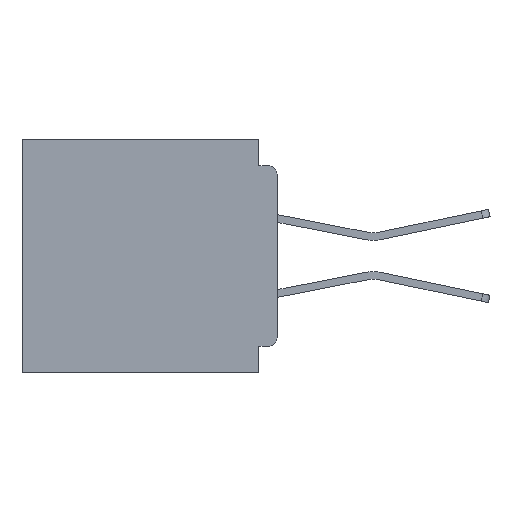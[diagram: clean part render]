
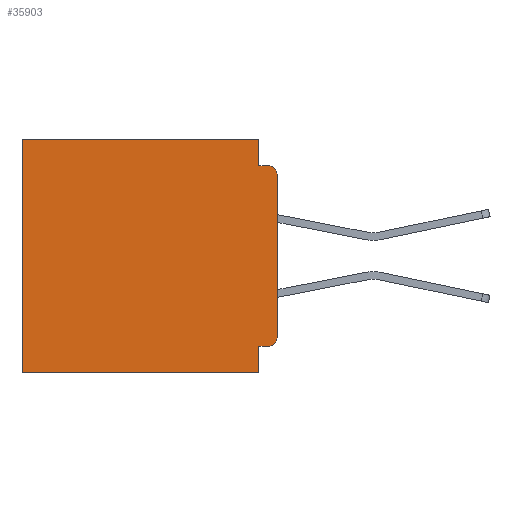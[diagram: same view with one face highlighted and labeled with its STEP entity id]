
A CAD part, left-side view. The second image highlights one B-rep face of the part: STEP entity #35903.
In plain terms, the highlighted planar face has unit normal (-1, 0, 0).
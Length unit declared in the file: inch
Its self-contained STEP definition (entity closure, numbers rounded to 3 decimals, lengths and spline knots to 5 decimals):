
#287 = ORIENTED_EDGE ( 'NONE', *, *, #53311, .F. ) ;
#643 = LINE ( 'NONE', #13273, #45786 ) ;
#1736 = DIRECTION ( 'NONE',  ( -1., 0., 0. ) ) ;
#2024 = ORIENTED_EDGE ( 'NONE', *, *, #27397, .T. ) ;
#2442 = ORIENTED_EDGE ( 'NONE', *, *, #39021, .F. ) ;
#3430 = ORIENTED_EDGE ( 'NONE', *, *, #11149, .F. ) ;
#4966 = DIRECTION ( 'NONE',  ( 1., 0., 0. ) ) ;
#5450 = VERTEX_POINT ( 'NONE', #17939 ) ;
#6329 = LINE ( 'NONE', #23212, #28919 ) ;
#6462 = VERTEX_POINT ( 'NONE', #16828 ) ;
#8554 = CARTESIAN_POINT ( 'NONE',  ( 0.3, 0.031, -0.4 ) ) ;
#8872 = CARTESIAN_POINT ( 'NONE',  ( 0.3, 0.015, -0.355 ) ) ;
#10659 = CARTESIAN_POINT ( 'NONE',  ( 0.3, 0.015, -0.34 ) ) ;
#10939 = VECTOR ( 'NONE', #56302, 39.37008 ) ;
#11149 = EDGE_CURVE ( 'NONE', #5450, #20077, #643, .T. ) ;
#11377 = VERTEX_POINT ( 'NONE', #20409 ) ;
#12421 = CARTESIAN_POINT ( 'NONE',  ( 0.3, 0., 0. ) ) ;
#13273 = CARTESIAN_POINT ( 'NONE',  ( 0.3, 0., -0.045 ) ) ;
#13822 = VERTEX_POINT ( 'NONE', #39043 ) ;
#15207 = DIRECTION ( 'NONE',  ( 0., 0., -1. ) ) ;
#15295 = CARTESIAN_POINT ( 'NONE',  ( 0.3, 0.437, -0.4 ) ) ;
#15383 = CIRCLE ( 'NONE', #31666, 0.015 ) ;
#16828 = CARTESIAN_POINT ( 'NONE',  ( 0.3, 0.031, -0.355 ) ) ;
#17407 = DIRECTION ( 'NONE',  ( 0., 0., -1. ) ) ;
#17939 = CARTESIAN_POINT ( 'NONE',  ( 0.3, 0.031, -0.045 ) ) ;
#18220 = VERTEX_POINT ( 'NONE', #47209 ) ;
#20077 = VERTEX_POINT ( 'NONE', #42108 ) ;
#20409 = CARTESIAN_POINT ( 'NONE',  ( 0.3, 0.437, 0. ) ) ;
#21222 = DIRECTION ( 'NONE',  ( 0., 0., -1. ) ) ;
#21391 = EDGE_CURVE ( 'NONE', #55388, #13822, #15383, .T. ) ;
#21596 = CIRCLE ( 'NONE', #55136, 0.015 ) ;
#22090 = VERTEX_POINT ( 'NONE', #56476 ) ;
#22447 = VECTOR ( 'NONE', #38396, 39.37008 ) ;
#22654 = ORIENTED_EDGE ( 'NONE', *, *, #26228, .T. ) ;
#22966 = PLANE ( 'NONE',  #56887 ) ;
#23001 = LINE ( 'NONE', #25025, #10939 ) ;
#23212 = CARTESIAN_POINT ( 'NONE',  ( 0.3, 0.031, 0. ) ) ;
#25025 = CARTESIAN_POINT ( 'NONE',  ( 0.3, 0., -0.355 ) ) ;
#25908 = ORIENTED_EDGE ( 'NONE', *, *, #29643, .T. ) ;
#26228 = EDGE_CURVE ( 'NONE', #11377, #55833, #51909, .T. ) ;
#26665 = VECTOR ( 'NONE', #42253, 39.37008 ) ;
#27397 = EDGE_CURVE ( 'NONE', #18220, #20077, #21596, .T. ) ;
#27709 = DIRECTION ( 'NONE',  ( 0., 0., -1. ) ) ;
#28153 = EDGE_LOOP ( 'NONE', ( #287, #2024, #3430, #35075, #25908, #22654, #2442, #57286, #47861, #32467 ) ) ;
#28797 = CARTESIAN_POINT ( 'NONE',  ( 0.3, 0.015, -0.06 ) ) ;
#28919 = VECTOR ( 'NONE', #27709, 39.37008 ) ;
#29050 = VECTOR ( 'NONE', #39421, 39.37008 ) ;
#29643 = EDGE_CURVE ( 'NONE', #22090, #11377, #40988, .T. ) ;
#31666 = AXIS2_PLACEMENT_3D ( 'NONE', #10659, #42159, #15207 ) ;
#31965 = CARTESIAN_POINT ( 'NONE',  ( 0.3, 0., -0.4 ) ) ;
#32467 = ORIENTED_EDGE ( 'NONE', *, *, #21391, .T. ) ;
#33273 = DIRECTION ( 'NONE',  ( 0., 0., -1. ) ) ;
#33843 = FACE_OUTER_BOUND ( 'NONE', #28153, .T. ) ;
#33865 = CARTESIAN_POINT ( 'NONE',  ( 0.3, 0., -0.4 ) ) ;
#35075 = ORIENTED_EDGE ( 'NONE', *, *, #50254, .F. ) ;
#35872 = VECTOR ( 'NONE', #21222, 39.37008 ) ;
#35903 = ADVANCED_FACE ( 'NONE', ( #33843 ), #22966, .F. ) ;
#36463 = DIRECTION ( 'NONE',  ( 0., 0., -1. ) ) ;
#38396 = DIRECTION ( 'NONE',  ( 0., 1., 0. ) ) ;
#39021 = EDGE_CURVE ( 'NONE', #54670, #55833, #56691, .T. ) ;
#39043 = CARTESIAN_POINT ( 'NONE',  ( 0.3, 0., -0.34 ) ) ;
#39421 = DIRECTION ( 'NONE',  ( 0., 1., 0. ) ) ;
#40459 = VECTOR ( 'NONE', #17407, 39.37008 ) ;
#40988 = LINE ( 'NONE', #12421, #29050 ) ;
#42108 = CARTESIAN_POINT ( 'NONE',  ( 0.3, 0.015, -0.045 ) ) ;
#42159 = DIRECTION ( 'NONE',  ( -1., 0., 0. ) ) ;
#42253 = DIRECTION ( 'NONE',  ( 0., 0., -1. ) ) ;
#44292 = EDGE_CURVE ( 'NONE', #6462, #54670, #47844, .T. ) ;
#44349 = CARTESIAN_POINT ( 'NONE',  ( 0.3, 0., -0.4 ) ) ;
#45487 = EDGE_CURVE ( 'NONE', #55388, #6462, #23001, .T. ) ;
#45786 = VECTOR ( 'NONE', #49294, 39.37008 ) ;
#47209 = CARTESIAN_POINT ( 'NONE',  ( 0.3, 0., -0.06 ) ) ;
#47844 = LINE ( 'NONE', #57003, #35872 ) ;
#47861 = ORIENTED_EDGE ( 'NONE', *, *, #45487, .F. ) ;
#49294 = DIRECTION ( 'NONE',  ( 0., -1., 0. ) ) ;
#50254 = EDGE_CURVE ( 'NONE', #22090, #5450, #6329, .T. ) ;
#51909 = LINE ( 'NONE', #15295, #26665 ) ;
#52340 = LINE ( 'NONE', #44349, #40459 ) ;
#52609 = CARTESIAN_POINT ( 'NONE',  ( 0.3, 0.437, -0.4 ) ) ;
#53311 = EDGE_CURVE ( 'NONE', #18220, #13822, #52340, .T. ) ;
#54670 = VERTEX_POINT ( 'NONE', #8554 ) ;
#55136 = AXIS2_PLACEMENT_3D ( 'NONE', #28797, #1736, #33273 ) ;
#55388 = VERTEX_POINT ( 'NONE', #8872 ) ;
#55833 = VERTEX_POINT ( 'NONE', #52609 ) ;
#56302 = DIRECTION ( 'NONE',  ( 0., 1., 0. ) ) ;
#56476 = CARTESIAN_POINT ( 'NONE',  ( 0.3, 0.031, 0. ) ) ;
#56691 = LINE ( 'NONE', #33865, #22447 ) ;
#56887 = AXIS2_PLACEMENT_3D ( 'NONE', #31965, #4966, #36463 ) ;
#57003 = CARTESIAN_POINT ( 'NONE',  ( 0.3, 0.031, -0.4 ) ) ;
#57286 = ORIENTED_EDGE ( 'NONE', *, *, #44292, .F. ) ;
